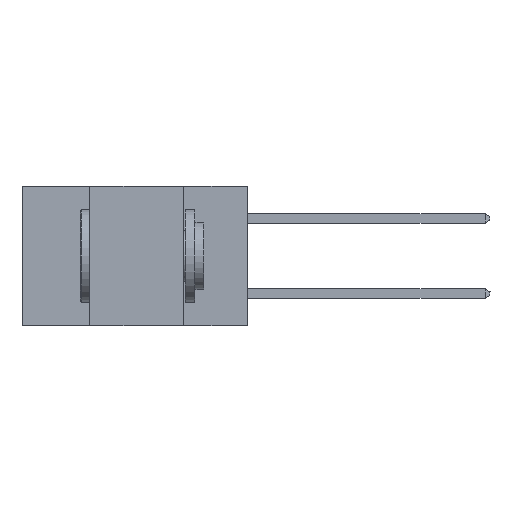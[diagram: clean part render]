
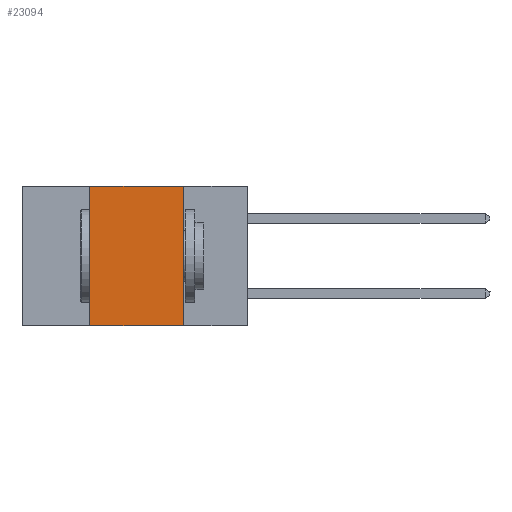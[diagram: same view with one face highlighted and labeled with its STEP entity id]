
A CAD part, left-side view. The second image highlights one B-rep face of the part: STEP entity #23094.
In plain terms, the highlighted planar face has unit normal (-1, 0, 0).
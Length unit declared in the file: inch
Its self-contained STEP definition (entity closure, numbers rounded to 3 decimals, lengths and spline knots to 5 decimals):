
#873 = ORIENTED_EDGE ( 'NONE', *, *, #22195, .F. ) ;
#2137 = LINE ( 'NONE', #13523, #20863 ) ;
#2950 = DIRECTION ( 'NONE',  ( 0., -1., 0. ) ) ;
#3268 = LINE ( 'NONE', #8137, #12666 ) ;
#4807 = CARTESIAN_POINT ( 'NONE',  ( 0., 0.6, -0.37 ) ) ;
#5806 = ORIENTED_EDGE ( 'NONE', *, *, #15041, .F. ) ;
#5902 = LINE ( 'NONE', #15129, #15353 ) ;
#6252 = DIRECTION ( 'NONE',  ( 0., 0., 1. ) ) ;
#6501 = CARTESIAN_POINT ( 'NONE',  ( 0., 0.6, 0. ) ) ;
#7784 = DIRECTION ( 'NONE',  ( 0., -1., 0. ) ) ;
#8032 = CARTESIAN_POINT ( 'NONE',  ( 0., 0.17, -0.37 ) ) ;
#8137 = CARTESIAN_POINT ( 'NONE',  ( 0., 0.42, -0.37 ) ) ;
#8380 = CARTESIAN_POINT ( 'NONE',  ( 0., 0.42, -0.37 ) ) ;
#8389 = PLANE ( 'NONE',  #20097 ) ;
#9247 = VERTEX_POINT ( 'NONE', #8380 ) ;
#10271 = EDGE_LOOP ( 'NONE', ( #873, #5806, #20765, #11425 ) ) ;
#10897 = FACE_OUTER_BOUND ( 'NONE', #10271, .T. ) ;
#11425 = ORIENTED_EDGE ( 'NONE', *, *, #14620, .T. ) ;
#11879 = VERTEX_POINT ( 'NONE', #12006 ) ;
#12006 = CARTESIAN_POINT ( 'NONE',  ( 0., 0.17, 0. ) ) ;
#12220 = DIRECTION ( 'NONE',  ( 0., 0., -1. ) ) ;
#12666 = VECTOR ( 'NONE', #6252, 39.37008 ) ;
#13523 = CARTESIAN_POINT ( 'NONE',  ( 0., 0.6, 0. ) ) ;
#14568 = VECTOR ( 'NONE', #2950, 39.37008 ) ;
#14620 = EDGE_CURVE ( 'NONE', #9247, #20250, #15146, .T. ) ;
#15041 = EDGE_CURVE ( 'NONE', #22716, #11879, #2137, .T. ) ;
#15129 = CARTESIAN_POINT ( 'NONE',  ( 0., 0.17, -0.37 ) ) ;
#15146 = LINE ( 'NONE', #4807, #14568 ) ;
#15353 = VECTOR ( 'NONE', #17039, 39.37008 ) ;
#17039 = DIRECTION ( 'NONE',  ( 0., 0., -1. ) ) ;
#20097 = AXIS2_PLACEMENT_3D ( 'NONE', #6501, #23382, #12220 ) ;
#20250 = VERTEX_POINT ( 'NONE', #8032 ) ;
#20765 = ORIENTED_EDGE ( 'NONE', *, *, #23009, .F. ) ;
#20863 = VECTOR ( 'NONE', #7784, 39.37008 ) ;
#22195 = EDGE_CURVE ( 'NONE', #11879, #20250, #5902, .T. ) ;
#22347 = CARTESIAN_POINT ( 'NONE',  ( 0., 0.42, 0. ) ) ;
#22716 = VERTEX_POINT ( 'NONE', #22347 ) ;
#23009 = EDGE_CURVE ( 'NONE', #9247, #22716, #3268, .T. ) ;
#23094 = ADVANCED_FACE ( 'NONE', ( #10897 ), #8389, .F. ) ;
#23382 = DIRECTION ( 'NONE',  ( 1., 0., 0. ) ) ;
